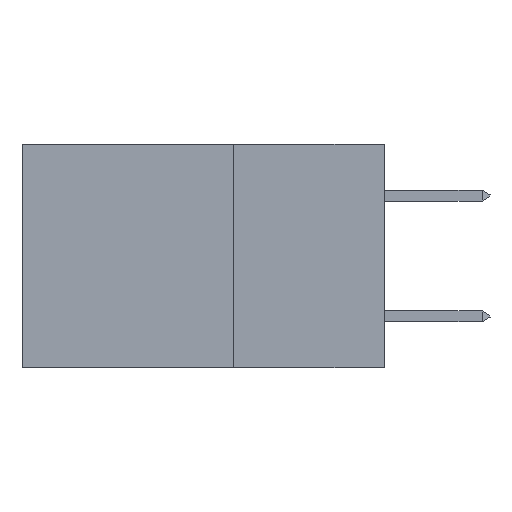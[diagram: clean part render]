
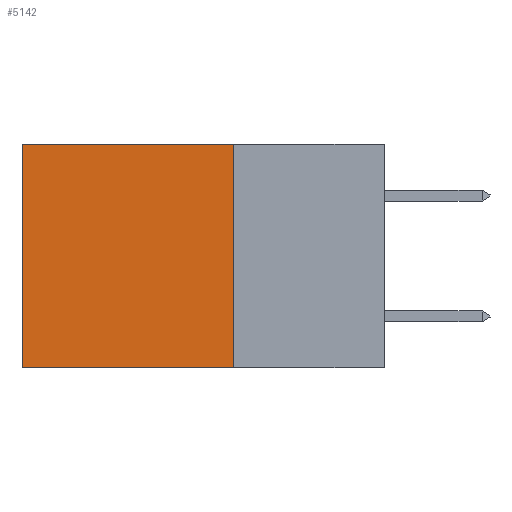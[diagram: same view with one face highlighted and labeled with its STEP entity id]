
A CAD part, left-side view. The second image highlights one B-rep face of the part: STEP entity #5142.
In plain terms, the highlighted planar face has unit normal (-1, 0, 0).
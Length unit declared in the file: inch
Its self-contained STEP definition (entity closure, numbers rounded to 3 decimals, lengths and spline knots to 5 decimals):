
#728 = CARTESIAN_POINT ( 'NONE',  ( 0.2875, 0.25, 0. ) ) ;
#1070 = DIRECTION ( 'NONE',  ( 1., 0., 0. ) ) ;
#2742 = VECTOR ( 'NONE', #9326, 39.37008 ) ;
#5142 = ADVANCED_FACE ( 'NONE', ( #40115 ), #20871, .F. ) ;
#7310 = CARTESIAN_POINT ( 'NONE',  ( 0.2875, 0.6, -0.37 ) ) ;
#7768 = AXIS2_PLACEMENT_3D ( 'NONE', #34874, #1070, #24712 ) ;
#8298 = EDGE_LOOP ( 'NONE', ( #17597, #40176, #23261, #33434 ) ) ;
#8639 = VECTOR ( 'NONE', #40580, 39.37008 ) ;
#9326 = DIRECTION ( 'NONE',  ( 0., 1., 0. ) ) ;
#10872 = EDGE_CURVE ( 'NONE', #15699, #35498, #24017, .T. ) ;
#11404 = EDGE_CURVE ( 'NONE', #15699, #14677, #22409, .T. ) ;
#14677 = VERTEX_POINT ( 'NONE', #39721 ) ;
#15362 = DIRECTION ( 'NONE',  ( 0., 0., -1. ) ) ;
#15699 = VERTEX_POINT ( 'NONE', #728 ) ;
#16447 = DIRECTION ( 'NONE',  ( 0., 1., 0. ) ) ;
#17597 = ORIENTED_EDGE ( 'NONE', *, *, #24536, .T. ) ;
#18730 = CARTESIAN_POINT ( 'NONE',  ( 0.2875, 0.25, 0. ) ) ;
#20871 = PLANE ( 'NONE',  #7768 ) ;
#22409 = LINE ( 'NONE', #18730, #25580 ) ;
#23261 = ORIENTED_EDGE ( 'NONE', *, *, #11404, .F. ) ;
#23796 = EDGE_CURVE ( 'NONE', #14677, #39993, #41664, .T. ) ;
#24017 = LINE ( 'NONE', #32962, #24571 ) ;
#24536 = EDGE_CURVE ( 'NONE', #35498, #39993, #26547, .T. ) ;
#24571 = VECTOR ( 'NONE', #16447, 39.37008 ) ;
#24712 = DIRECTION ( 'NONE',  ( 0., 0., -1. ) ) ;
#25580 = VECTOR ( 'NONE', #15362, 39.37008 ) ;
#26547 = LINE ( 'NONE', #40300, #8639 ) ;
#30096 = CARTESIAN_POINT ( 'NONE',  ( 0.2875, 0.6, 0. ) ) ;
#32962 = CARTESIAN_POINT ( 'NONE',  ( 0.2875, 0.25, 0. ) ) ;
#33028 = CARTESIAN_POINT ( 'NONE',  ( 0.2875, 0.25, -0.37 ) ) ;
#33434 = ORIENTED_EDGE ( 'NONE', *, *, #10872, .T. ) ;
#34874 = CARTESIAN_POINT ( 'NONE',  ( 0.2875, 0.25, 0. ) ) ;
#35498 = VERTEX_POINT ( 'NONE', #30096 ) ;
#39721 = CARTESIAN_POINT ( 'NONE',  ( 0.2875, 0.25, -0.37 ) ) ;
#39993 = VERTEX_POINT ( 'NONE', #7310 ) ;
#40115 = FACE_OUTER_BOUND ( 'NONE', #8298, .T. ) ;
#40176 = ORIENTED_EDGE ( 'NONE', *, *, #23796, .F. ) ;
#40300 = CARTESIAN_POINT ( 'NONE',  ( 0.2875, 0.6, 0. ) ) ;
#40580 = DIRECTION ( 'NONE',  ( 0., 0., -1. ) ) ;
#41664 = LINE ( 'NONE', #33028, #2742 ) ;
